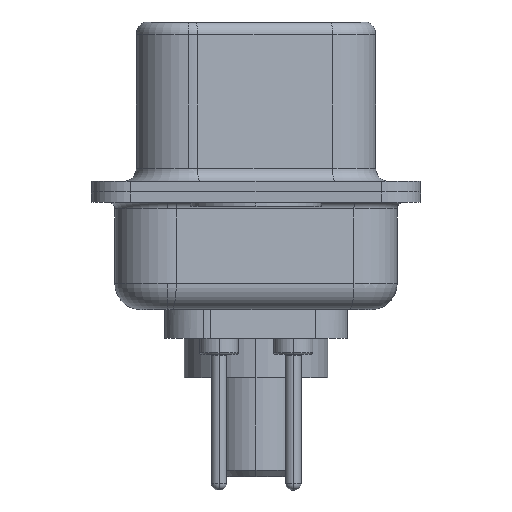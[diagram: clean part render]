
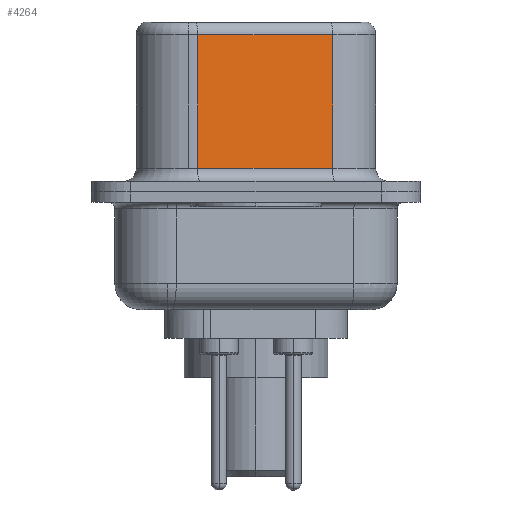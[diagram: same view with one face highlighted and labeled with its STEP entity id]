
A CAD part, left-side view. The second image highlights one B-rep face of the part: STEP entity #4264.
In plain terms, the highlighted planar face has unit normal (-0.985, -0.174, 0).
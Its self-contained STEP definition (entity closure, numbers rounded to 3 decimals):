
#608 = VERTEX_POINT ( 'NONE', #1632 ) ;
#899 = EDGE_CURVE ( 'NONE', #8767, #608, #8675, .T. ) ;
#951 = FACE_OUTER_BOUND ( 'NONE', #8220, .T. ) ;
#1297 = CARTESIAN_POINT ( 'NONE',  ( 4.58, -2.927, 6.02 ) ) ;
#1377 = LINE ( 'NONE', #5194, #8491 ) ;
#1593 = DIRECTION ( 'NONE',  ( 0.985, 0.174, 0. ) ) ;
#1630 = VECTOR ( 'NONE', #11581, 1000. ) ;
#1632 = CARTESIAN_POINT ( 'NONE',  ( 3.67, 2.233, 0.9 ) ) ;
#1930 = LINE ( 'NONE', #1297, #1630 ) ;
#2854 = LINE ( 'NONE', #10293, #7572 ) ;
#3434 = CARTESIAN_POINT ( 'NONE',  ( 4.58, -2.927, 6.52 ) ) ;
#3520 = EDGE_CURVE ( 'NONE', #608, #9410, #2854, .T. ) ;
#3600 = DIRECTION ( 'NONE',  ( 0.174, -0.985, 0. ) ) ;
#4264 = ADVANCED_FACE ( 'NONE', ( #951 ), #6276, .F. ) ;
#4433 = CARTESIAN_POINT ( 'NONE',  ( 3.67, 2.233, 6.02 ) ) ;
#4928 = ORIENTED_EDGE ( 'NONE', *, *, #3520, .T. ) ;
#5194 = CARTESIAN_POINT ( 'NONE',  ( 4.58, -2.927, 6.52 ) ) ;
#5199 = AXIS2_PLACEMENT_3D ( 'NONE', #3434, #1593, #8193 ) ;
#5463 = CARTESIAN_POINT ( 'NONE',  ( 4.58, -2.927, 6.02 ) ) ;
#6276 = PLANE ( 'NONE',  #5199 ) ;
#6735 = EDGE_CURVE ( 'NONE', #7634, #8767, #1930, .T. ) ;
#6807 = ORIENTED_EDGE ( 'NONE', *, *, #9307, .F. ) ;
#7572 = VECTOR ( 'NONE', #3600, 1000. ) ;
#7634 = VERTEX_POINT ( 'NONE', #5463 ) ;
#8182 = ORIENTED_EDGE ( 'NONE', *, *, #899, .T. ) ;
#8193 = DIRECTION ( 'NONE',  ( -0.174, 0.985, 0. ) ) ;
#8220 = EDGE_LOOP ( 'NONE', ( #6807, #10449, #8182, #4928 ) ) ;
#8392 = VECTOR ( 'NONE', #10171, 1000. ) ;
#8491 = VECTOR ( 'NONE', #10843, 1000. ) ;
#8675 = LINE ( 'NONE', #11304, #8392 ) ;
#8767 = VERTEX_POINT ( 'NONE', #4433 ) ;
#9307 = EDGE_CURVE ( 'NONE', #7634, #9410, #1377, .T. ) ;
#9410 = VERTEX_POINT ( 'NONE', #10037 ) ;
#10037 = CARTESIAN_POINT ( 'NONE',  ( 4.58, -2.927, 0.9 ) ) ;
#10171 = DIRECTION ( 'NONE',  ( 0., 0., -1. ) ) ;
#10293 = CARTESIAN_POINT ( 'NONE',  ( 4.58, -2.927, 0.9 ) ) ;
#10449 = ORIENTED_EDGE ( 'NONE', *, *, #6735, .T. ) ;
#10843 = DIRECTION ( 'NONE',  ( 0., 0., -1. ) ) ;
#11304 = CARTESIAN_POINT ( 'NONE',  ( 3.67, 2.233, 6.52 ) ) ;
#11581 = DIRECTION ( 'NONE',  ( -0.174, 0.985, 0. ) ) ;
